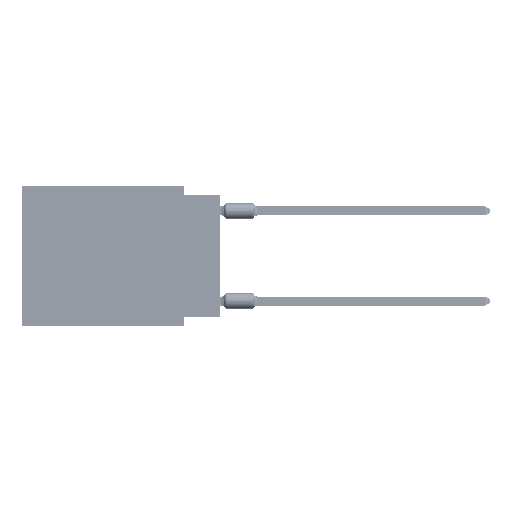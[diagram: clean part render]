
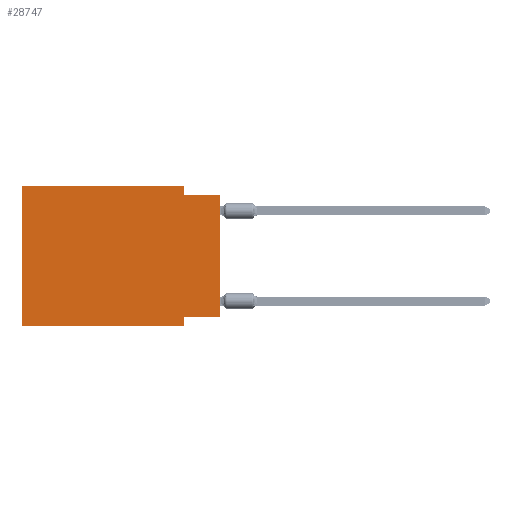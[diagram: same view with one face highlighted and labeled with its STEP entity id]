
A CAD part, left-side view. The second image highlights one B-rep face of the part: STEP entity #28747.
In plain terms, the highlighted planar face has unit normal (-1, 0, 0).
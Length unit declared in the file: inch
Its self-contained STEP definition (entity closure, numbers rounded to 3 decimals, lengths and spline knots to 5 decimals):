
#246 = LINE ( 'NONE', #36674, #40331 ) ;
#2802 = VECTOR ( 'NONE', #64268, 39.37008 ) ;
#3015 = EDGE_CURVE ( 'NONE', #9294, #33081, #64648, .T. ) ;
#3355 = CARTESIAN_POINT ( 'NONE',  ( 0., 0.1, -0.365 ) ) ;
#6756 = VERTEX_POINT ( 'NONE', #13551 ) ;
#7043 = ORIENTED_EDGE ( 'NONE', *, *, #19265, .F. ) ;
#7650 = ORIENTED_EDGE ( 'NONE', *, *, #55581, .F. ) ;
#7968 = FACE_OUTER_BOUND ( 'NONE', #30119, .T. ) ;
#9294 = VERTEX_POINT ( 'NONE', #36423 ) ;
#10962 = DIRECTION ( 'NONE',  ( 0., -1., 0. ) ) ;
#11159 = VECTOR ( 'NONE', #41938, 39.37008 ) ;
#12744 = CARTESIAN_POINT ( 'NONE',  ( 0., 0.1, -0.39 ) ) ;
#13043 = EDGE_CURVE ( 'NONE', #38601, #17009, #54013, .T. ) ;
#13444 = LINE ( 'NONE', #54582, #56308 ) ;
#13551 = CARTESIAN_POINT ( 'NONE',  ( 0., 0.1, 0. ) ) ;
#17009 = VERTEX_POINT ( 'NONE', #61307 ) ;
#18763 = VERTEX_POINT ( 'NONE', #3355 ) ;
#19265 = EDGE_CURVE ( 'NONE', #6756, #38601, #69834, .T. ) ;
#21908 = EDGE_CURVE ( 'NONE', #21974, #18763, #13444, .T. ) ;
#21974 = VERTEX_POINT ( 'NONE', #74911 ) ;
#22450 = CARTESIAN_POINT ( 'NONE',  ( 0., 0.1, 0. ) ) ;
#24483 = LINE ( 'NONE', #12744, #72711 ) ;
#27621 = ORIENTED_EDGE ( 'NONE', *, *, #54433, .F. ) ;
#28747 = ADVANCED_FACE ( 'NONE', ( #7968 ), #32228, .F. ) ;
#29111 = DIRECTION ( 'NONE',  ( 0., 0., -1. ) ) ;
#29712 = ORIENTED_EDGE ( 'NONE', *, *, #68877, .F. ) ;
#30119 = EDGE_LOOP ( 'NONE', ( #47004, #41977, #7043, #27621, #29712, #40334, #7650, #71548 ) ) ;
#32228 = PLANE ( 'NONE',  #56461 ) ;
#33081 = VERTEX_POINT ( 'NONE', #43710 ) ;
#34874 = CARTESIAN_POINT ( 'NONE',  ( 0., 0., 0. ) ) ;
#36397 = CARTESIAN_POINT ( 'NONE',  ( 0., 0., -0.025 ) ) ;
#36423 = CARTESIAN_POINT ( 'NONE',  ( 0., 0.55, -0.39 ) ) ;
#36674 = CARTESIAN_POINT ( 'NONE',  ( 0., 0.55, 0. ) ) ;
#36964 = CARTESIAN_POINT ( 'NONE',  ( 0., 0.55, 0. ) ) ;
#37741 = DIRECTION ( 'NONE',  ( 1., 0., 0. ) ) ;
#37953 = CARTESIAN_POINT ( 'NONE',  ( 0., 0.1, -0.025 ) ) ;
#38601 = VERTEX_POINT ( 'NONE', #37953 ) ;
#40331 = VECTOR ( 'NONE', #71926, 39.37008 ) ;
#40334 = ORIENTED_EDGE ( 'NONE', *, *, #3015, .T. ) ;
#41938 = DIRECTION ( 'NONE',  ( 0., 0., 1. ) ) ;
#41977 = ORIENTED_EDGE ( 'NONE', *, *, #13043, .F. ) ;
#42514 = DIRECTION ( 'NONE',  ( 0., 0., -1. ) ) ;
#43592 = VECTOR ( 'NONE', #72415, 39.37008 ) ;
#43710 = CARTESIAN_POINT ( 'NONE',  ( 0., 0.1, -0.39 ) ) ;
#46026 = EDGE_CURVE ( 'NONE', #21974, #17009, #59147, .T. ) ;
#47004 = ORIENTED_EDGE ( 'NONE', *, *, #46026, .T. ) ;
#51326 = CARTESIAN_POINT ( 'NONE',  ( 0., 0.55, 0. ) ) ;
#54013 = LINE ( 'NONE', #36397, #43592 ) ;
#54433 = EDGE_CURVE ( 'NONE', #54441, #6756, #57597, .T. ) ;
#54441 = VERTEX_POINT ( 'NONE', #64221 ) ;
#54582 = CARTESIAN_POINT ( 'NONE',  ( 0., 0., -0.365 ) ) ;
#55581 = EDGE_CURVE ( 'NONE', #18763, #33081, #24483, .T. ) ;
#56308 = VECTOR ( 'NONE', #61599, 39.37008 ) ;
#56461 = AXIS2_PLACEMENT_3D ( 'NONE', #36964, #37741, #60842 ) ;
#57597 = LINE ( 'NONE', #51326, #58811 ) ;
#58811 = VECTOR ( 'NONE', #10962, 39.37008 ) ;
#59147 = LINE ( 'NONE', #34874, #11159 ) ;
#60842 = DIRECTION ( 'NONE',  ( 0., 0., -1. ) ) ;
#61307 = CARTESIAN_POINT ( 'NONE',  ( 0., 0., -0.025 ) ) ;
#61599 = DIRECTION ( 'NONE',  ( 0., 1., 0. ) ) ;
#64221 = CARTESIAN_POINT ( 'NONE',  ( 0., 0.55, 0. ) ) ;
#64268 = DIRECTION ( 'NONE',  ( 0., -1., 0. ) ) ;
#64648 = LINE ( 'NONE', #71327, #2802 ) ;
#67452 = VECTOR ( 'NONE', #29111, 39.37008 ) ;
#68877 = EDGE_CURVE ( 'NONE', #9294, #54441, #246, .T. ) ;
#69834 = LINE ( 'NONE', #22450, #67452 ) ;
#71327 = CARTESIAN_POINT ( 'NONE',  ( 0., 0.55, -0.39 ) ) ;
#71548 = ORIENTED_EDGE ( 'NONE', *, *, #21908, .F. ) ;
#71926 = DIRECTION ( 'NONE',  ( 0., 0., 1. ) ) ;
#72415 = DIRECTION ( 'NONE',  ( 0., -1., 0. ) ) ;
#72711 = VECTOR ( 'NONE', #42514, 39.37008 ) ;
#74911 = CARTESIAN_POINT ( 'NONE',  ( 0., 0., -0.365 ) ) ;
